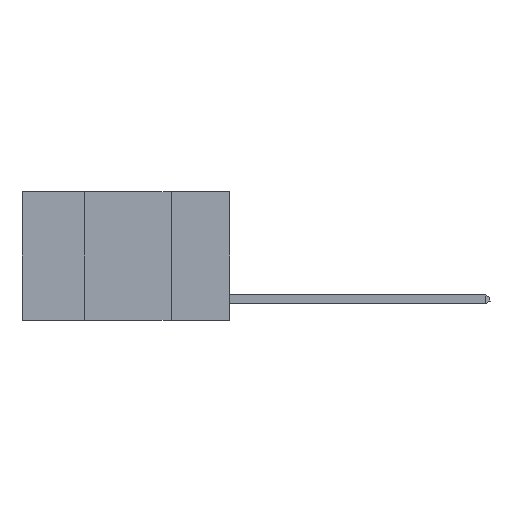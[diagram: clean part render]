
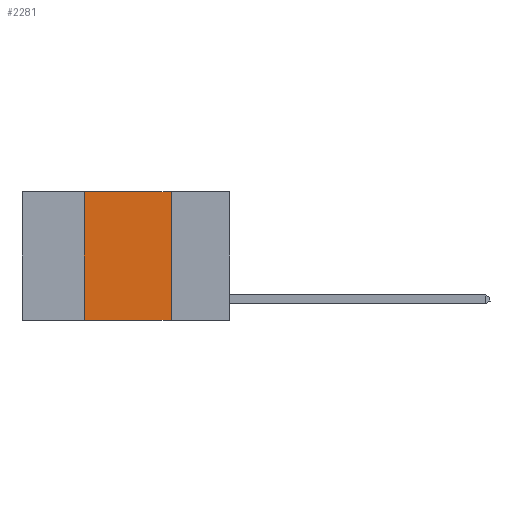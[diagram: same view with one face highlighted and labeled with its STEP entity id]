
A CAD part, left-side view. The second image highlights one B-rep face of the part: STEP entity #2281.
In plain terms, the highlighted planar face has unit normal (-1, 0, 0).
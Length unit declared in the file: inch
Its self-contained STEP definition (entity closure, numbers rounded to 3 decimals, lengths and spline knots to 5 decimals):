
#301 = ORIENTED_EDGE ( 'NONE', *, *, #12227, .F. ) ;
#345 = PLANE ( 'NONE',  #7856 ) ;
#834 = VECTOR ( 'NONE', #12425, 39.37008 ) ;
#1503 = DIRECTION ( 'NONE',  ( 0., 0., -1. ) ) ;
#1646 = CARTESIAN_POINT ( 'NONE',  ( 0., 0.42, 0. ) ) ;
#1757 = CARTESIAN_POINT ( 'NONE',  ( 0., 0.6, 0. ) ) ;
#2281 = ADVANCED_FACE ( 'NONE', ( #8172 ), #345, .F. ) ;
#2557 = CARTESIAN_POINT ( 'NONE',  ( 0., 0.42, 0. ) ) ;
#3093 = VERTEX_POINT ( 'NONE', #4832 ) ;
#3853 = LINE ( 'NONE', #7173, #6981 ) ;
#3916 = CARTESIAN_POINT ( 'NONE',  ( 0., 0.6, 0. ) ) ;
#3972 = ORIENTED_EDGE ( 'NONE', *, *, #15122, .F. ) ;
#4062 = DIRECTION ( 'NONE',  ( 0., 0., -1. ) ) ;
#4832 = CARTESIAN_POINT ( 'NONE',  ( 0., 0.17, 0. ) ) ;
#4885 = EDGE_CURVE ( 'NONE', #13367, #11008, #12404, .T. ) ;
#5048 = EDGE_CURVE ( 'NONE', #13367, #9233, #5355, .T. ) ;
#5086 = DIRECTION ( 'NONE',  ( 1., 0., 0. ) ) ;
#5355 = LINE ( 'NONE', #12697, #834 ) ;
#6860 = LINE ( 'NONE', #1757, #9839 ) ;
#6880 = CARTESIAN_POINT ( 'NONE',  ( 0., 0.42, -0.37 ) ) ;
#6981 = VECTOR ( 'NONE', #1503, 39.37008 ) ;
#7173 = CARTESIAN_POINT ( 'NONE',  ( 0., 0.17, 0. ) ) ;
#7174 = CARTESIAN_POINT ( 'NONE',  ( 0., 0.17, -0.37 ) ) ;
#7542 = DIRECTION ( 'NONE',  ( 0., 0., 1. ) ) ;
#7856 = AXIS2_PLACEMENT_3D ( 'NONE', #3916, #5086, #4062 ) ;
#8172 = FACE_OUTER_BOUND ( 'NONE', #11234, .T. ) ;
#9233 = VERTEX_POINT ( 'NONE', #7174 ) ;
#9466 = VECTOR ( 'NONE', #7542, 39.37008 ) ;
#9839 = VECTOR ( 'NONE', #14734, 39.37008 ) ;
#11008 = VERTEX_POINT ( 'NONE', #2557 ) ;
#11234 = EDGE_LOOP ( 'NONE', ( #3972, #301, #12132, #12832 ) ) ;
#12132 = ORIENTED_EDGE ( 'NONE', *, *, #4885, .F. ) ;
#12227 = EDGE_CURVE ( 'NONE', #11008, #3093, #6860, .T. ) ;
#12404 = LINE ( 'NONE', #1646, #9466 ) ;
#12425 = DIRECTION ( 'NONE',  ( 0., -1., 0. ) ) ;
#12697 = CARTESIAN_POINT ( 'NONE',  ( 0., 0.6, -0.37 ) ) ;
#12832 = ORIENTED_EDGE ( 'NONE', *, *, #5048, .T. ) ;
#13367 = VERTEX_POINT ( 'NONE', #6880 ) ;
#14734 = DIRECTION ( 'NONE',  ( 0., -1., 0. ) ) ;
#15122 = EDGE_CURVE ( 'NONE', #3093, #9233, #3853, .T. ) ;
